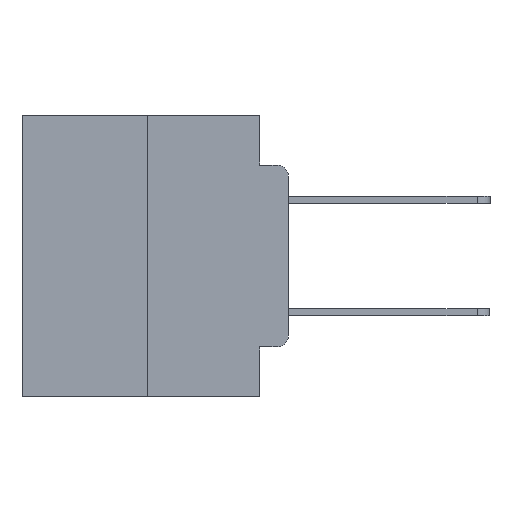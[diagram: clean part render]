
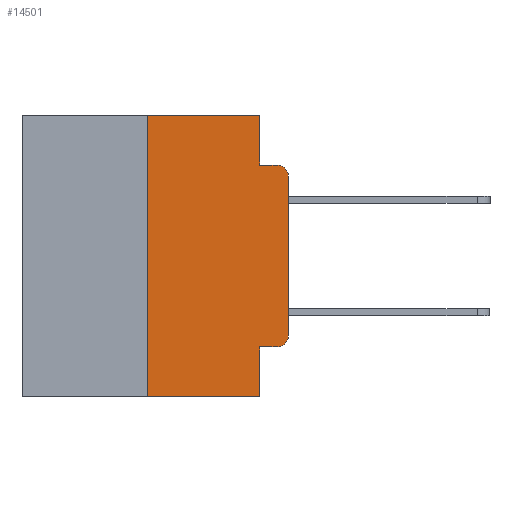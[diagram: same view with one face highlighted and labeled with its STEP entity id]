
A CAD part, left-side view. The second image highlights one B-rep face of the part: STEP entity #14501.
In plain terms, the highlighted planar face has unit normal (-1, 0, 0).
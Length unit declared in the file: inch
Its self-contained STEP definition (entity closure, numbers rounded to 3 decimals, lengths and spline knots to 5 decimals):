
#64 = VERTEX_POINT ( 'NONE', #8882 ) ;
#190 = VERTEX_POINT ( 'NONE', #14960 ) ;
#201 = AXIS2_PLACEMENT_3D ( 'NONE', #6756, #21129, #8802 ) ;
#271 = VERTEX_POINT ( 'NONE', #6821 ) ;
#356 = ORIENTED_EDGE ( 'NONE', *, *, #7007, .F. ) ;
#781 = VERTEX_POINT ( 'NONE', #22043 ) ;
#913 = CARTESIAN_POINT ( 'NONE',  ( 0., 0.051, -0.0885 ) ) ;
#1168 = EDGE_CURVE ( 'NONE', #271, #15984, #10455, .T. ) ;
#1234 = VECTOR ( 'NONE', #8656, 39.37008 ) ;
#1595 = ORIENTED_EDGE ( 'NONE', *, *, #7357, .T. ) ;
#1952 = LINE ( 'NONE', #16928, #1234 ) ;
#2149 = CARTESIAN_POINT ( 'NONE',  ( 0., 0.473, 0. ) ) ;
#2204 = DIRECTION ( 'NONE',  ( 0., 0., -1. ) ) ;
#2464 = DIRECTION ( 'NONE',  ( 1., 0., 0. ) ) ;
#2678 = EDGE_CURVE ( 'NONE', #16831, #20669, #9196, .T. ) ;
#2690 = CARTESIAN_POINT ( 'NONE',  ( 0., 0.02, -0.1085 ) ) ;
#3464 = ORIENTED_EDGE ( 'NONE', *, *, #1168, .F. ) ;
#3510 = AXIS2_PLACEMENT_3D ( 'NONE', #2690, #17346, #4873 ) ;
#3688 = VERTEX_POINT ( 'NONE', #8875 ) ;
#4873 = DIRECTION ( 'NONE',  ( 0., 0., -1. ) ) ;
#5012 = CARTESIAN_POINT ( 'NONE',  ( 0., 0.25, 0. ) ) ;
#5055 = LINE ( 'NONE', #9090, #10579 ) ;
#5318 = DIRECTION ( 'NONE',  ( 0., -1., 0. ) ) ;
#6756 = CARTESIAN_POINT ( 'NONE',  ( 0., 0.02, -0.3915 ) ) ;
#6821 = CARTESIAN_POINT ( 'NONE',  ( 0., 0.051, -0.4115 ) ) ;
#7007 = EDGE_CURVE ( 'NONE', #64, #14176, #5055, .T. ) ;
#7331 = ORIENTED_EDGE ( 'NONE', *, *, #15828, .T. ) ;
#7357 = EDGE_CURVE ( 'NONE', #16831, #15984, #1952, .T. ) ;
#7855 = FACE_OUTER_BOUND ( 'NONE', #26283, .T. ) ;
#7867 = CARTESIAN_POINT ( 'NONE',  ( 0., 0.051, -0.4115 ) ) ;
#8115 = AXIS2_PLACEMENT_3D ( 'NONE', #15031, #2464, #17124 ) ;
#8498 = VERTEX_POINT ( 'NONE', #10418 ) ;
#8656 = DIRECTION ( 'NONE',  ( 0., -1., 0. ) ) ;
#8802 = DIRECTION ( 'NONE',  ( 0., 0., -1. ) ) ;
#8817 = LINE ( 'NONE', #913, #19176 ) ;
#8875 = CARTESIAN_POINT ( 'NONE',  ( 0., 0., -0.3915 ) ) ;
#8882 = CARTESIAN_POINT ( 'NONE',  ( 0., 0.051, 0. ) ) ;
#9090 = CARTESIAN_POINT ( 'NONE',  ( 0., 0.051, 0. ) ) ;
#9118 = LINE ( 'NONE', #2149, #12664 ) ;
#9196 = LINE ( 'NONE', #17752, #18911 ) ;
#9625 = CARTESIAN_POINT ( 'NONE',  ( 0., 0., 0. ) ) ;
#9736 = VECTOR ( 'NONE', #21940, 39.37008 ) ;
#9777 = CARTESIAN_POINT ( 'NONE',  ( 0., 0.051, -0.0885 ) ) ;
#9820 = DIRECTION ( 'NONE',  ( 0., 0., 1. ) ) ;
#10256 = CIRCLE ( 'NONE', #3510, 0.02 ) ;
#10418 = CARTESIAN_POINT ( 'NONE',  ( 0., 0., -0.1085 ) ) ;
#10455 = LINE ( 'NONE', #19967, #20736 ) ;
#10579 = VECTOR ( 'NONE', #21409, 39.37008 ) ;
#10856 = PLANE ( 'NONE',  #8115 ) ;
#10896 = VECTOR ( 'NONE', #14748, 39.37008 ) ;
#11142 = EDGE_CURVE ( 'NONE', #14176, #190, #8817, .T. ) ;
#11528 = ORIENTED_EDGE ( 'NONE', *, *, #15323, .T. ) ;
#12379 = CARTESIAN_POINT ( 'NONE',  ( 0., 0.25, -0.5 ) ) ;
#12664 = VECTOR ( 'NONE', #24971, 39.37008 ) ;
#13919 = EDGE_CURVE ( 'NONE', #8498, #190, #10256, .T. ) ;
#14176 = VERTEX_POINT ( 'NONE', #9777 ) ;
#14501 = ADVANCED_FACE ( 'NONE', ( #7855 ), #10856, .F. ) ;
#14748 = DIRECTION ( 'NONE',  ( 0., -1., 0. ) ) ;
#14960 = CARTESIAN_POINT ( 'NONE',  ( 0., 0.02, -0.0885 ) ) ;
#14993 = EDGE_CURVE ( 'NONE', #20669, #64, #9118, .T. ) ;
#15031 = CARTESIAN_POINT ( 'NONE',  ( 0., 0.473, 0. ) ) ;
#15323 = EDGE_CURVE ( 'NONE', #3688, #8498, #26104, .T. ) ;
#15828 = EDGE_CURVE ( 'NONE', #781, #3688, #21301, .T. ) ;
#15974 = ORIENTED_EDGE ( 'NONE', *, *, #14993, .F. ) ;
#15984 = VERTEX_POINT ( 'NONE', #25657 ) ;
#16295 = ORIENTED_EDGE ( 'NONE', *, *, #2678, .F. ) ;
#16418 = LINE ( 'NONE', #7867, #10896 ) ;
#16831 = VERTEX_POINT ( 'NONE', #12379 ) ;
#16928 = CARTESIAN_POINT ( 'NONE',  ( 0., 0.473, -0.5 ) ) ;
#17124 = DIRECTION ( 'NONE',  ( 0., 0., -1. ) ) ;
#17346 = DIRECTION ( 'NONE',  ( -1., 0., 0. ) ) ;
#17752 = CARTESIAN_POINT ( 'NONE',  ( 0., 0.25, 0. ) ) ;
#18603 = EDGE_CURVE ( 'NONE', #271, #781, #16418, .T. ) ;
#18851 = ORIENTED_EDGE ( 'NONE', *, *, #11142, .F. ) ;
#18911 = VECTOR ( 'NONE', #9820, 39.37008 ) ;
#19176 = VECTOR ( 'NONE', #5318, 39.37008 ) ;
#19967 = CARTESIAN_POINT ( 'NONE',  ( 0., 0.051, 0. ) ) ;
#20669 = VERTEX_POINT ( 'NONE', #5012 ) ;
#20736 = VECTOR ( 'NONE', #2204, 39.37008 ) ;
#21129 = DIRECTION ( 'NONE',  ( -1., 0., 0. ) ) ;
#21301 = CIRCLE ( 'NONE', #201, 0.02 ) ;
#21409 = DIRECTION ( 'NONE',  ( 0., 0., -1. ) ) ;
#21940 = DIRECTION ( 'NONE',  ( 0., 0., 1. ) ) ;
#22023 = ORIENTED_EDGE ( 'NONE', *, *, #13919, .T. ) ;
#22043 = CARTESIAN_POINT ( 'NONE',  ( 0., 0.02, -0.4115 ) ) ;
#23149 = ORIENTED_EDGE ( 'NONE', *, *, #18603, .T. ) ;
#24971 = DIRECTION ( 'NONE',  ( 0., -1., 0. ) ) ;
#25657 = CARTESIAN_POINT ( 'NONE',  ( 0., 0.051, -0.5 ) ) ;
#26104 = LINE ( 'NONE', #9625, #9736 ) ;
#26283 = EDGE_LOOP ( 'NONE', ( #11528, #22023, #18851, #356, #15974, #16295, #1595, #3464, #23149, #7331 ) ) ;
